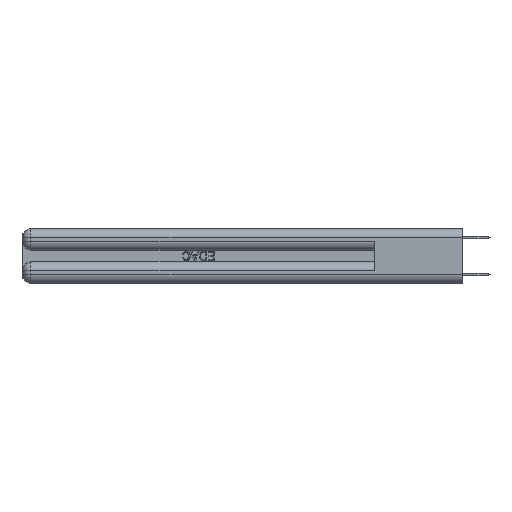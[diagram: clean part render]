
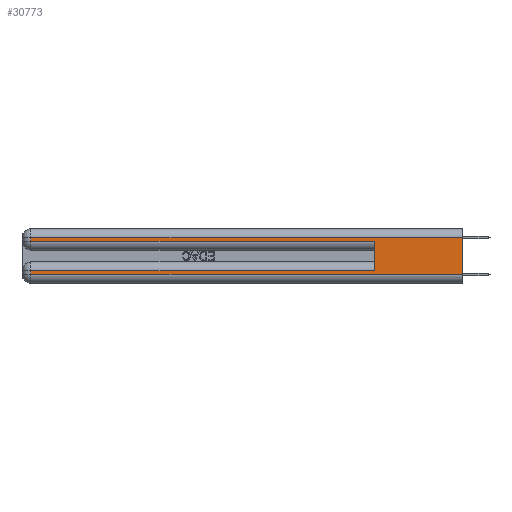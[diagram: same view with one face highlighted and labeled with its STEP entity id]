
A CAD part, left-side view. The second image highlights one B-rep face of the part: STEP entity #30773.
In plain terms, the highlighted planar face has unit normal (-1, 0, 0).
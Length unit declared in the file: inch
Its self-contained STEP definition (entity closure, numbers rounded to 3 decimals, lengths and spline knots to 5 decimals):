
#1185 = VERTEX_POINT ( 'NONE', #7527 ) ;
#1330 = VERTEX_POINT ( 'NONE', #34504 ) ;
#1381 = DIRECTION ( 'NONE',  ( 0., -1., 0. ) ) ;
#2026 = CARTESIAN_POINT ( 'NONE',  ( 0., 0.6, 0.285 ) ) ;
#2541 = DIRECTION ( 'NONE',  ( 0., 0., -1. ) ) ;
#2584 = CARTESIAN_POINT ( 'NONE',  ( 0., 0., 0.37 ) ) ;
#2715 = FACE_OUTER_BOUND ( 'NONE', #9392, .T. ) ;
#3248 = LINE ( 'NONE', #25014, #20451 ) ;
#3360 = ORIENTED_EDGE ( 'NONE', *, *, #34683, .T. ) ;
#4004 = CARTESIAN_POINT ( 'NONE',  ( 0., 0.6, 0.145 ) ) ;
#4006 = VECTOR ( 'NONE', #20784, 39.37008 ) ;
#4579 = ORIENTED_EDGE ( 'NONE', *, *, #20034, .F. ) ;
#4688 = DIRECTION ( 'NONE',  ( 0., 1., 0. ) ) ;
#6644 = CARTESIAN_POINT ( 'NONE',  ( 0., 0., 0.285 ) ) ;
#7424 = EDGE_CURVE ( 'NONE', #31784, #18117, #34730, .T. ) ;
#7527 = CARTESIAN_POINT ( 'NONE',  ( 0., 0.6, 0.085 ) ) ;
#7535 = VECTOR ( 'NONE', #23239, 39.37008 ) ;
#7569 = DIRECTION ( 'NONE',  ( 0., 0., -1. ) ) ;
#7793 = LINE ( 'NONE', #26913, #13327 ) ;
#8344 = VERTEX_POINT ( 'NONE', #18312 ) ;
#9392 = EDGE_LOOP ( 'NONE', ( #4579, #28272, #22472, #33701, #31650, #3360, #30907, #29534 ) ) ;
#9664 = VERTEX_POINT ( 'NONE', #11751 ) ;
#9863 = VECTOR ( 'NONE', #1381, 39.37008 ) ;
#10060 = EDGE_CURVE ( 'NONE', #1185, #21650, #15047, .T. ) ;
#10942 = LINE ( 'NONE', #2584, #26168 ) ;
#11070 = PLANE ( 'NONE',  #27498 ) ;
#11751 = CARTESIAN_POINT ( 'NONE',  ( 0., 2.94, 0.085 ) ) ;
#11870 = LINE ( 'NONE', #28479, #9863 ) ;
#13327 = VECTOR ( 'NONE', #34952, 39.37008 ) ;
#13562 = CARTESIAN_POINT ( 'NONE',  ( 0., 0., 0.37 ) ) ;
#15047 = LINE ( 'NONE', #4004, #4006 ) ;
#15083 = VECTOR ( 'NONE', #7569, 39.37008 ) ;
#18117 = VERTEX_POINT ( 'NONE', #26544 ) ;
#18312 = CARTESIAN_POINT ( 'NONE',  ( 0., 0., 0.31 ) ) ;
#19656 = DIRECTION ( 'NONE',  ( 0., 0., -1. ) ) ;
#20034 = EDGE_CURVE ( 'NONE', #8344, #1330, #10942, .T. ) ;
#20451 = VECTOR ( 'NONE', #19656, 39.37008 ) ;
#20784 = DIRECTION ( 'NONE',  ( 0., 0., 1. ) ) ;
#21650 = VERTEX_POINT ( 'NONE', #2026 ) ;
#22472 = ORIENTED_EDGE ( 'NONE', *, *, #7424, .T. ) ;
#23239 = DIRECTION ( 'NONE',  ( 0., -1., 0. ) ) ;
#24545 = EDGE_CURVE ( 'NONE', #18117, #21650, #31463, .T. ) ;
#25014 = CARTESIAN_POINT ( 'NONE',  ( 0., 2.94, 0.37 ) ) ;
#25158 = CARTESIAN_POINT ( 'NONE',  ( 0., 2.94, 0.31 ) ) ;
#26168 = VECTOR ( 'NONE', #27205, 39.37008 ) ;
#26278 = EDGE_CURVE ( 'NONE', #9664, #33751, #3248, .T. ) ;
#26544 = CARTESIAN_POINT ( 'NONE',  ( 0., 2.94, 0.285 ) ) ;
#26631 = CARTESIAN_POINT ( 'NONE',  ( 0., 0., 0.31 ) ) ;
#26913 = CARTESIAN_POINT ( 'NONE',  ( 0., 0., 0.085 ) ) ;
#27205 = DIRECTION ( 'NONE',  ( 0., 0., -1. ) ) ;
#27498 = AXIS2_PLACEMENT_3D ( 'NONE', #13562, #35017, #2541 ) ;
#28272 = ORIENTED_EDGE ( 'NONE', *, *, #30585, .T. ) ;
#28479 = CARTESIAN_POINT ( 'NONE',  ( 0., 0., 0.06 ) ) ;
#28951 = LINE ( 'NONE', #26631, #30920 ) ;
#29534 = ORIENTED_EDGE ( 'NONE', *, *, #33735, .T. ) ;
#30585 = EDGE_CURVE ( 'NONE', #8344, #31784, #28951, .T. ) ;
#30773 = ADVANCED_FACE ( 'NONE', ( #2715 ), #11070, .F. ) ;
#30907 = ORIENTED_EDGE ( 'NONE', *, *, #26278, .T. ) ;
#30920 = VECTOR ( 'NONE', #4688, 39.37008 ) ;
#31463 = LINE ( 'NONE', #6644, #7535 ) ;
#31650 = ORIENTED_EDGE ( 'NONE', *, *, #10060, .F. ) ;
#31784 = VERTEX_POINT ( 'NONE', #25158 ) ;
#32042 = CARTESIAN_POINT ( 'NONE',  ( 0., 2.94, 0.37 ) ) ;
#33516 = CARTESIAN_POINT ( 'NONE',  ( 0., 2.94, 0.06 ) ) ;
#33701 = ORIENTED_EDGE ( 'NONE', *, *, #24545, .T. ) ;
#33735 = EDGE_CURVE ( 'NONE', #33751, #1330, #11870, .T. ) ;
#33751 = VERTEX_POINT ( 'NONE', #33516 ) ;
#34504 = CARTESIAN_POINT ( 'NONE',  ( 0., 0., 0.06 ) ) ;
#34683 = EDGE_CURVE ( 'NONE', #1185, #9664, #7793, .T. ) ;
#34730 = LINE ( 'NONE', #32042, #15083 ) ;
#34952 = DIRECTION ( 'NONE',  ( 0., 1., 0. ) ) ;
#35017 = DIRECTION ( 'NONE',  ( 1., 0., 0. ) ) ;
